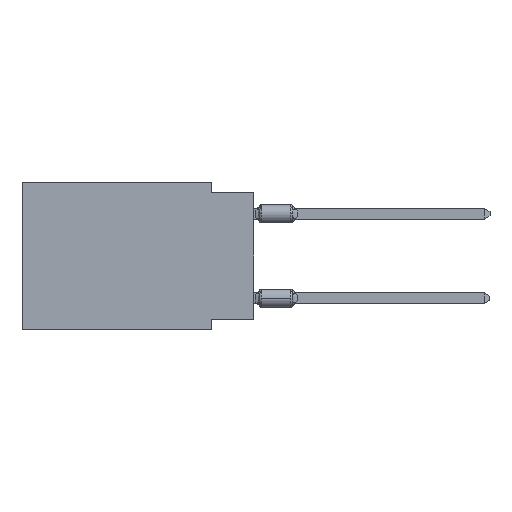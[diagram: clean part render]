
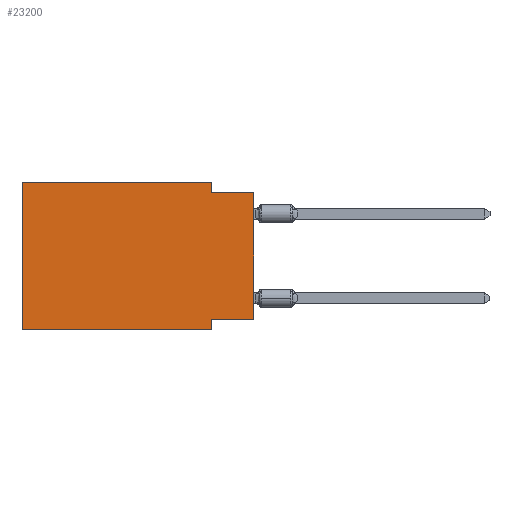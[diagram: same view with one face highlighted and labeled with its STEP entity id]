
A CAD part, left-side view. The second image highlights one B-rep face of the part: STEP entity #23200.
In plain terms, the highlighted planar face has unit normal (-1, 0, 0).
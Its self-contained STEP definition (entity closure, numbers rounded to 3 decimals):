
#106 = CARTESIAN_POINT ( 'NONE',  ( 0., 13.97, -8.89 ) ) ;
#199 = EDGE_CURVE ( 'NONE', #24952, #11387, #27989, .T. ) ;
#620 = VECTOR ( 'NONE', #12193, 1000. ) ;
#737 = CARTESIAN_POINT ( 'NONE',  ( 0., 13.97, 0. ) ) ;
#762 = VECTOR ( 'NONE', #5014, 1000. ) ;
#808 = CARTESIAN_POINT ( 'NONE',  ( 0., 2.54, -8.255 ) ) ;
#1431 = CARTESIAN_POINT ( 'NONE',  ( 0., 0., -8.255 ) ) ;
#1474 = VERTEX_POINT ( 'NONE', #808 ) ;
#1786 = VERTEX_POINT ( 'NONE', #10882 ) ;
#2193 = FACE_OUTER_BOUND ( 'NONE', #6548, .T. ) ;
#2258 = CARTESIAN_POINT ( 'NONE',  ( 0., 0., -0.635 ) ) ;
#2726 = DIRECTION ( 'NONE',  ( 0., -1., 0. ) ) ;
#3027 = CARTESIAN_POINT ( 'NONE',  ( 0., 2.54, -8.89 ) ) ;
#3389 = VECTOR ( 'NONE', #3470, 1000. ) ;
#3470 = DIRECTION ( 'NONE',  ( 0., 0., -1. ) ) ;
#3997 = VERTEX_POINT ( 'NONE', #4008 ) ;
#4008 = CARTESIAN_POINT ( 'NONE',  ( 0., 2.54, 0. ) ) ;
#4889 = ORIENTED_EDGE ( 'NONE', *, *, #8428, .F. ) ;
#5014 = DIRECTION ( 'NONE',  ( 0., -1., 0. ) ) ;
#5297 = CARTESIAN_POINT ( 'NONE',  ( 0., 0., 0. ) ) ;
#5474 = CARTESIAN_POINT ( 'NONE',  ( 0., 0., -8.255 ) ) ;
#5501 = EDGE_CURVE ( 'NONE', #3997, #1786, #20707, .T. ) ;
#6206 = CARTESIAN_POINT ( 'NONE',  ( 0., 13.97, 0. ) ) ;
#6548 = EDGE_LOOP ( 'NONE', ( #6598, #26828, #27618, #15129, #4889, #16571, #19025, #24679 ) ) ;
#6598 = ORIENTED_EDGE ( 'NONE', *, *, #199, .T. ) ;
#8428 = EDGE_CURVE ( 'NONE', #12470, #19942, #26266, .T. ) ;
#9199 = VECTOR ( 'NONE', #21013, 1000. ) ;
#9531 = VERTEX_POINT ( 'NONE', #3027 ) ;
#9591 = VECTOR ( 'NONE', #2726, 1000. ) ;
#10205 = DIRECTION ( 'NONE',  ( 0., 1., 0. ) ) ;
#10882 = CARTESIAN_POINT ( 'NONE',  ( 0., 2.54, -0.635 ) ) ;
#11387 = VERTEX_POINT ( 'NONE', #21993 ) ;
#12193 = DIRECTION ( 'NONE',  ( 0., 0., 1. ) ) ;
#12470 = VERTEX_POINT ( 'NONE', #106 ) ;
#13037 = VECTOR ( 'NONE', #10205, 1000. ) ;
#13698 = CARTESIAN_POINT ( 'NONE',  ( 0., 13.97, -8.89 ) ) ;
#14156 = EDGE_CURVE ( 'NONE', #24952, #1474, #23521, .T. ) ;
#15129 = ORIENTED_EDGE ( 'NONE', *, *, #22652, .F. ) ;
#15645 = DIRECTION ( 'NONE',  ( 1., 0., 0. ) ) ;
#16571 = ORIENTED_EDGE ( 'NONE', *, *, #27320, .T. ) ;
#17091 = EDGE_CURVE ( 'NONE', #1474, #9531, #25711, .T. ) ;
#19025 = ORIENTED_EDGE ( 'NONE', *, *, #17091, .F. ) ;
#19522 = VECTOR ( 'NONE', #24182, 1000. ) ;
#19942 = VERTEX_POINT ( 'NONE', #737 ) ;
#20707 = LINE ( 'NONE', #25696, #9199 ) ;
#20867 = LINE ( 'NONE', #13698, #9591 ) ;
#21013 = DIRECTION ( 'NONE',  ( 0., 0., -1. ) ) ;
#21167 = CARTESIAN_POINT ( 'NONE',  ( 0., 2.54, -8.89 ) ) ;
#21360 = EDGE_CURVE ( 'NONE', #1786, #11387, #22295, .T. ) ;
#21993 = CARTESIAN_POINT ( 'NONE',  ( 0., 0., -0.635 ) ) ;
#22090 = DIRECTION ( 'NONE',  ( 0., 0., -1. ) ) ;
#22295 = LINE ( 'NONE', #2258, #762 ) ;
#22652 = EDGE_CURVE ( 'NONE', #19942, #3997, #28143, .T. ) ;
#23063 = CARTESIAN_POINT ( 'NONE',  ( 0., 13.97, 0. ) ) ;
#23200 = ADVANCED_FACE ( 'NONE', ( #2193 ), #26626, .F. ) ;
#23363 = DIRECTION ( 'NONE',  ( 0., 0., 1. ) ) ;
#23521 = LINE ( 'NONE', #1431, #13037 ) ;
#24034 = CARTESIAN_POINT ( 'NONE',  ( 0., 13.97, 0. ) ) ;
#24182 = DIRECTION ( 'NONE',  ( 0., -1., 0. ) ) ;
#24679 = ORIENTED_EDGE ( 'NONE', *, *, #14156, .F. ) ;
#24952 = VERTEX_POINT ( 'NONE', #5474 ) ;
#25696 = CARTESIAN_POINT ( 'NONE',  ( 0., 2.54, 0. ) ) ;
#25711 = LINE ( 'NONE', #21167, #3389 ) ;
#26088 = AXIS2_PLACEMENT_3D ( 'NONE', #23063, #15645, #22090 ) ;
#26266 = LINE ( 'NONE', #6206, #28047 ) ;
#26626 = PLANE ( 'NONE',  #26088 ) ;
#26828 = ORIENTED_EDGE ( 'NONE', *, *, #21360, .F. ) ;
#27320 = EDGE_CURVE ( 'NONE', #12470, #9531, #20867, .T. ) ;
#27618 = ORIENTED_EDGE ( 'NONE', *, *, #5501, .F. ) ;
#27989 = LINE ( 'NONE', #5297, #620 ) ;
#28047 = VECTOR ( 'NONE', #23363, 1000. ) ;
#28143 = LINE ( 'NONE', #24034, #19522 ) ;
